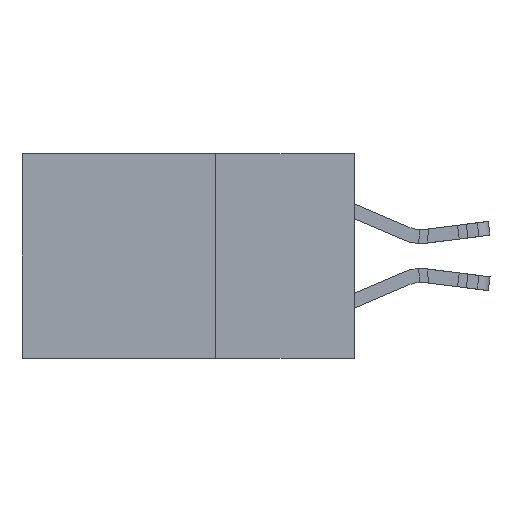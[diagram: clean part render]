
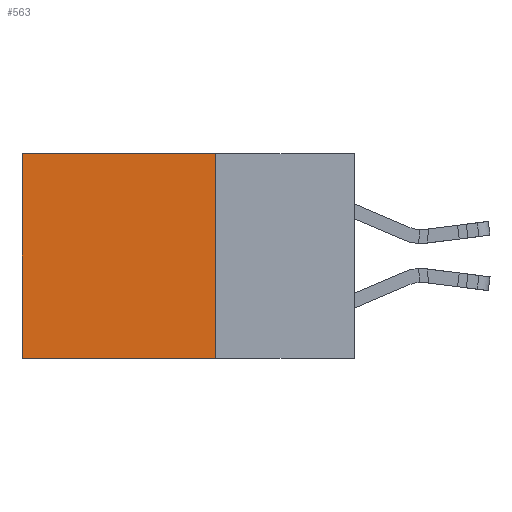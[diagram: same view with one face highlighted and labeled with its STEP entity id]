
A CAD part, left-side view. The second image highlights one B-rep face of the part: STEP entity #563.
In plain terms, the highlighted planar face has unit normal (-1, 0, 0).
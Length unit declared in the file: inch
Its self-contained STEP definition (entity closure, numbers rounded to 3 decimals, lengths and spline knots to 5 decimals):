
#563 = ADVANCED_FACE ( 'NONE', ( #29091 ), #17988, .F. ) ;
#912 = LINE ( 'NONE', #1764, #24294 ) ;
#982 = AXIS2_PLACEMENT_3D ( 'NONE', #12675, #7856, #15602 ) ;
#1764 = CARTESIAN_POINT ( 'NONE',  ( 0.298, 0.25, 0. ) ) ;
#1768 = ORIENTED_EDGE ( 'NONE', *, *, #32642, .F. ) ;
#1839 = LINE ( 'NONE', #9023, #2279 ) ;
#2279 = VECTOR ( 'NONE', #27644, 39.37008 ) ;
#4852 = LINE ( 'NONE', #28534, #17737 ) ;
#7856 = DIRECTION ( 'NONE',  ( 1., 0., 0. ) ) ;
#9023 = CARTESIAN_POINT ( 'NONE',  ( 0.298, 0.25, -0.37 ) ) ;
#10436 = DIRECTION ( 'NONE',  ( 0., 0., -1. ) ) ;
#11482 = DIRECTION ( 'NONE',  ( 0., 0., -1. ) ) ;
#12036 = VERTEX_POINT ( 'NONE', #31018 ) ;
#12675 = CARTESIAN_POINT ( 'NONE',  ( 0.298, 0.25, 0. ) ) ;
#13171 = VERTEX_POINT ( 'NONE', #17968 ) ;
#14400 = CARTESIAN_POINT ( 'NONE',  ( 0.298, 0.6, -0.37 ) ) ;
#14878 = EDGE_LOOP ( 'NONE', ( #26100, #21616, #1768, #26336 ) ) ;
#15602 = DIRECTION ( 'NONE',  ( 0., 0., -1. ) ) ;
#17737 = VECTOR ( 'NONE', #31224, 39.37008 ) ;
#17968 = CARTESIAN_POINT ( 'NONE',  ( 0.298, 0.6, 0. ) ) ;
#17988 = PLANE ( 'NONE',  #982 ) ;
#18492 = LINE ( 'NONE', #30897, #29795 ) ;
#20735 = VERTEX_POINT ( 'NONE', #30103 ) ;
#20814 = EDGE_CURVE ( 'NONE', #13171, #23551, #18492, .T. ) ;
#21616 = ORIENTED_EDGE ( 'NONE', *, *, #27968, .F. ) ;
#23551 = VERTEX_POINT ( 'NONE', #14400 ) ;
#24294 = VECTOR ( 'NONE', #11482, 39.37008 ) ;
#25168 = EDGE_CURVE ( 'NONE', #20735, #13171, #4852, .T. ) ;
#26100 = ORIENTED_EDGE ( 'NONE', *, *, #20814, .T. ) ;
#26336 = ORIENTED_EDGE ( 'NONE', *, *, #25168, .T. ) ;
#27644 = DIRECTION ( 'NONE',  ( 0., 1., 0. ) ) ;
#27968 = EDGE_CURVE ( 'NONE', #12036, #23551, #1839, .T. ) ;
#28534 = CARTESIAN_POINT ( 'NONE',  ( 0.298, 0.25, 0. ) ) ;
#29091 = FACE_OUTER_BOUND ( 'NONE', #14878, .T. ) ;
#29795 = VECTOR ( 'NONE', #10436, 39.37008 ) ;
#30103 = CARTESIAN_POINT ( 'NONE',  ( 0.298, 0.25, 0. ) ) ;
#30897 = CARTESIAN_POINT ( 'NONE',  ( 0.298, 0.6, 0. ) ) ;
#31018 = CARTESIAN_POINT ( 'NONE',  ( 0.298, 0.25, -0.37 ) ) ;
#31224 = DIRECTION ( 'NONE',  ( 0., 1., 0. ) ) ;
#32642 = EDGE_CURVE ( 'NONE', #20735, #12036, #912, .T. ) ;
